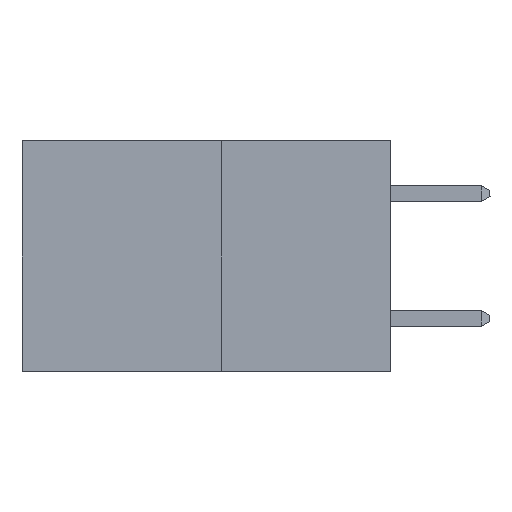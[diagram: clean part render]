
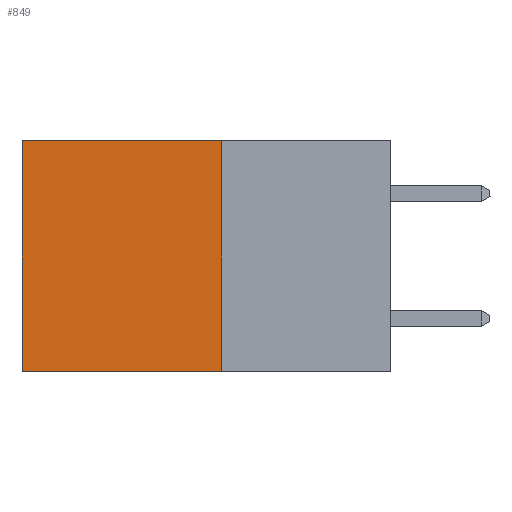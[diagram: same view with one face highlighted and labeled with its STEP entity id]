
A CAD part, left-side view. The second image highlights one B-rep face of the part: STEP entity #849.
In plain terms, the highlighted planar face has unit normal (-1, 0, 0).
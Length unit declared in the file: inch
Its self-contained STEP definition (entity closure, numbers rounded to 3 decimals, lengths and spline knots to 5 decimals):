
#849 = ADVANCED_FACE ( 'NONE', ( #9797 ), #16247, .F. ) ;
#1033 = LINE ( 'NONE', #18733, #5879 ) ;
#1397 = VERTEX_POINT ( 'NONE', #16357 ) ;
#2531 = EDGE_CURVE ( 'NONE', #23215, #1397, #18945, .T. ) ;
#3114 = ORIENTED_EDGE ( 'NONE', *, *, #9438, .F. ) ;
#4331 = VERTEX_POINT ( 'NONE', #16207 ) ;
#4994 = EDGE_LOOP ( 'NONE', ( #12379, #5092, #3114, #23492 ) ) ;
#5092 = ORIENTED_EDGE ( 'NONE', *, *, #13533, .F. ) ;
#5879 = VECTOR ( 'NONE', #12684, 39.37008 ) ;
#6535 = CARTESIAN_POINT ( 'NONE',  ( 0.277, 0.59, 0. ) ) ;
#7354 = DIRECTION ( 'NONE',  ( 0., 1., 0. ) ) ;
#9438 = EDGE_CURVE ( 'NONE', #4331, #13456, #24469, .T. ) ;
#9489 = DIRECTION ( 'NONE',  ( 0., 0., -1. ) ) ;
#9557 = CARTESIAN_POINT ( 'NONE',  ( 0.277, 0.27, -0.37 ) ) ;
#9797 = FACE_OUTER_BOUND ( 'NONE', #4994, .T. ) ;
#12379 = ORIENTED_EDGE ( 'NONE', *, *, #2531, .T. ) ;
#12421 = CARTESIAN_POINT ( 'NONE',  ( 0.277, 0.27, -0.37 ) ) ;
#12684 = DIRECTION ( 'NONE',  ( 0., 1., 0. ) ) ;
#12962 = VECTOR ( 'NONE', #22666, 39.37008 ) ;
#13456 = VERTEX_POINT ( 'NONE', #12421 ) ;
#13533 = EDGE_CURVE ( 'NONE', #13456, #1397, #1033, .T. ) ;
#13796 = VECTOR ( 'NONE', #9489, 39.37008 ) ;
#14703 = VECTOR ( 'NONE', #7354, 39.37008 ) ;
#14981 = DIRECTION ( 'NONE',  ( 0., 0., -1. ) ) ;
#16137 = DIRECTION ( 'NONE',  ( 1., 0., 0. ) ) ;
#16207 = CARTESIAN_POINT ( 'NONE',  ( 0.277, 0.27, 0. ) ) ;
#16247 = PLANE ( 'NONE',  #25537 ) ;
#16357 = CARTESIAN_POINT ( 'NONE',  ( 0.277, 0.59, -0.37 ) ) ;
#18733 = CARTESIAN_POINT ( 'NONE',  ( 0.277, 0.27, -0.37 ) ) ;
#18945 = LINE ( 'NONE', #22839, #12962 ) ;
#19497 = CARTESIAN_POINT ( 'NONE',  ( 0.277, 0.27, 0. ) ) ;
#22666 = DIRECTION ( 'NONE',  ( 0., 0., -1. ) ) ;
#22839 = CARTESIAN_POINT ( 'NONE',  ( 0.277, 0.59, -0.37 ) ) ;
#23215 = VERTEX_POINT ( 'NONE', #6535 ) ;
#23492 = ORIENTED_EDGE ( 'NONE', *, *, #26078, .T. ) ;
#23629 = CARTESIAN_POINT ( 'NONE',  ( 0.277, 0.27, -0.37 ) ) ;
#24469 = LINE ( 'NONE', #23629, #13796 ) ;
#25372 = LINE ( 'NONE', #19497, #14703 ) ;
#25537 = AXIS2_PLACEMENT_3D ( 'NONE', #9557, #16137, #14981 ) ;
#26078 = EDGE_CURVE ( 'NONE', #4331, #23215, #25372, .T. ) ;
